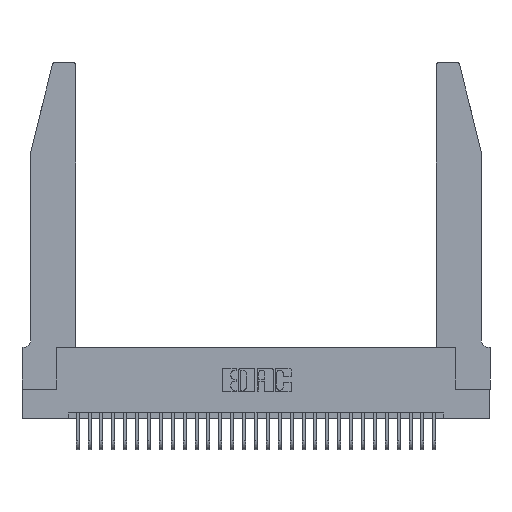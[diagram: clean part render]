
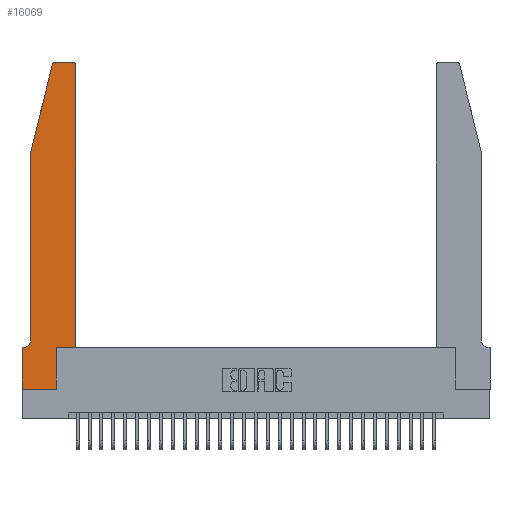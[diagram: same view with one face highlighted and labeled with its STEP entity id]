
A CAD part, top view. The second image highlights one B-rep face of the part: STEP entity #16069.
In plain terms, the highlighted planar face has unit normal (0, 0, 1).
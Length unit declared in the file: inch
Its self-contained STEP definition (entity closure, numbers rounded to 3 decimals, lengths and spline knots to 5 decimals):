
#297 = CARTESIAN_POINT ( 'NONE',  ( 0.4205, 2.72, 0.37 ) ) ;
#377 = EDGE_CURVE ( 'NONE', #8615, #3096, #2190, .T. ) ;
#385 = DIRECTION ( 'NONE',  ( 1., 0., 0. ) ) ;
#727 = EDGE_CURVE ( 'NONE', #26823, #5615, #28646, .T. ) ;
#1028 = EDGE_CURVE ( 'NONE', #5615, #10951, #1361, .T. ) ;
#1029 = CARTESIAN_POINT ( 'NONE',  ( 0.4505, 2.72, 0.37 ) ) ;
#1043 = VECTOR ( 'NONE', #2668, 39.37008 ) ;
#1126 = ORIENTED_EDGE ( 'NONE', *, *, #11851, .T. ) ;
#1361 = LINE ( 'NONE', #2361, #12913 ) ;
#1579 = EDGE_CURVE ( 'NONE', #10951, #21455, #11445, .T. ) ;
#1671 = CIRCLE ( 'NONE', #4736, 0.03 ) ;
#1751 = ORIENTED_EDGE ( 'NONE', *, *, #12945, .T. ) ;
#1956 = EDGE_LOOP ( 'NONE', ( #27631, #6244, #1751, #22483, #5915, #8851, #1126, #10419, #12542, #1984, #29123, #8060 ) ) ;
#1984 = ORIENTED_EDGE ( 'NONE', *, *, #727, .T. ) ;
#2190 = LINE ( 'NONE', #12530, #8380 ) ;
#2299 = VERTEX_POINT ( 'NONE', #7763 ) ;
#2361 = CARTESIAN_POINT ( 'NONE',  ( 0.4505, 0.35, 0.37 ) ) ;
#2425 = DIRECTION ( 'NONE',  ( 0., 0., -1. ) ) ;
#2523 = DIRECTION ( 'NONE',  ( 0., 1., 0. ) ) ;
#2608 = DIRECTION ( 'NONE',  ( 1., 0., 0. ) ) ;
#2668 = DIRECTION ( 'NONE',  ( -1., 0., 0. ) ) ;
#2748 = DIRECTION ( 'NONE',  ( 0., 0., 1. ) ) ;
#2757 = DIRECTION ( 'NONE',  ( 0., 1., 0. ) ) ;
#2860 = EDGE_CURVE ( 'NONE', #3096, #26823, #4192, .T. ) ;
#3047 = CARTESIAN_POINT ( 'NONE',  ( 0., 0.35, 0.37 ) ) ;
#3096 = VERTEX_POINT ( 'NONE', #26735 ) ;
#3155 = VECTOR ( 'NONE', #25083, 39.37008 ) ;
#3467 = CARTESIAN_POINT ( 'NONE',  ( 0.2865, 0.35, 0.37 ) ) ;
#3954 = LINE ( 'NONE', #26986, #15414 ) ;
#4134 = DIRECTION ( 'NONE',  ( 0., -1., 0. ) ) ;
#4192 = LINE ( 'NONE', #7428, #20300 ) ;
#4346 = CARTESIAN_POINT ( 'NONE',  ( 0., 0.35, 0.37 ) ) ;
#4482 = CARTESIAN_POINT ( 'NONE',  ( 0.2605, 2.75, 0.37 ) ) ;
#4736 = AXIS2_PLACEMENT_3D ( 'NONE', #16496, #2748, #18805 ) ;
#5313 = VECTOR ( 'NONE', #27944, 39.37008 ) ;
#5404 = VERTEX_POINT ( 'NONE', #3047 ) ;
#5615 = VERTEX_POINT ( 'NONE', #22076 ) ;
#5915 = ORIENTED_EDGE ( 'NONE', *, *, #7186, .T. ) ;
#6244 = ORIENTED_EDGE ( 'NONE', *, *, #22508, .T. ) ;
#6357 = DIRECTION ( 'NONE',  ( 0., -1., 0. ) ) ;
#6574 = EDGE_CURVE ( 'NONE', #11440, #5404, #14012, .T. ) ;
#7186 = EDGE_CURVE ( 'NONE', #2299, #11440, #21830, .T. ) ;
#7428 = CARTESIAN_POINT ( 'NONE',  ( 0.2865, 0.35, 0.37 ) ) ;
#7453 = CARTESIAN_POINT ( 'NONE',  ( 0.0755, 2., 0.37 ) ) ;
#7763 = CARTESIAN_POINT ( 'NONE',  ( 0.0755, 0.42, 0.37 ) ) ;
#8060 = ORIENTED_EDGE ( 'NONE', *, *, #1579, .T. ) ;
#8380 = VECTOR ( 'NONE', #385, 39.37008 ) ;
#8587 = FACE_OUTER_BOUND ( 'NONE', #1956, .T. ) ;
#8615 = VERTEX_POINT ( 'NONE', #10075 ) ;
#8851 = ORIENTED_EDGE ( 'NONE', *, *, #6574, .T. ) ;
#9110 = PLANE ( 'NONE',  #16142 ) ;
#9832 = CARTESIAN_POINT ( 'NONE',  ( 0.25487, 2.72718, 0.37 ) ) ;
#9971 = EDGE_CURVE ( 'NONE', #10111, #2299, #15187, .T. ) ;
#10066 = AXIS2_PLACEMENT_3D ( 'NONE', #16183, #2425, #18488 ) ;
#10075 = CARTESIAN_POINT ( 'NONE',  ( 0., 0., 0.37 ) ) ;
#10111 = VERTEX_POINT ( 'NONE', #13662 ) ;
#10419 = ORIENTED_EDGE ( 'NONE', *, *, #377, .T. ) ;
#10951 = VERTEX_POINT ( 'NONE', #1029 ) ;
#11294 = VECTOR ( 'NONE', #4134, 39.37008 ) ;
#11403 = DIRECTION ( 'NONE',  ( 0., 0., 1. ) ) ;
#11440 = VERTEX_POINT ( 'NONE', #14291 ) ;
#11445 = CIRCLE ( 'NONE', #16043, 0.03 ) ;
#11851 = EDGE_CURVE ( 'NONE', #5404, #8615, #3954, .T. ) ;
#12530 = CARTESIAN_POINT ( 'NONE',  ( 0., 0., 0.37 ) ) ;
#12542 = ORIENTED_EDGE ( 'NONE', *, *, #2860, .T. ) ;
#12600 = EDGE_CURVE ( 'NONE', #21455, #26869, #15356, .T. ) ;
#12913 = VECTOR ( 'NONE', #2523, 39.37008 ) ;
#12945 = EDGE_CURVE ( 'NONE', #21382, #10111, #23526, .T. ) ;
#13662 = CARTESIAN_POINT ( 'NONE',  ( 0.0755, 2., 0.37 ) ) ;
#14012 = LINE ( 'NONE', #21006, #1043 ) ;
#14291 = CARTESIAN_POINT ( 'NONE',  ( 0.0055, 0.35, 0.37 ) ) ;
#15187 = LINE ( 'NONE', #17863, #11294 ) ;
#15356 = LINE ( 'NONE', #4482, #3155 ) ;
#15414 = VECTOR ( 'NONE', #6357, 39.37008 ) ;
#15495 = CARTESIAN_POINT ( 'NONE',  ( 0.4505, 0.35, 0.37 ) ) ;
#16043 = AXIS2_PLACEMENT_3D ( 'NONE', #297, #16364, #2608 ) ;
#16069 = ADVANCED_FACE ( 'NONE', ( #8587 ), #9110, .T. ) ;
#16142 = AXIS2_PLACEMENT_3D ( 'NONE', #4346, #11403, #27275 ) ;
#16183 = CARTESIAN_POINT ( 'NONE',  ( 0.0055, 0.42, 0.37 ) ) ;
#16364 = DIRECTION ( 'NONE',  ( 0., 0., 1. ) ) ;
#16496 = CARTESIAN_POINT ( 'NONE',  ( 0.284, 2.72, 0.37 ) ) ;
#17863 = CARTESIAN_POINT ( 'NONE',  ( 0.0755, 2., 0.37 ) ) ;
#18488 = DIRECTION ( 'NONE',  ( -1., 0., 0. ) ) ;
#18805 = DIRECTION ( 'NONE',  ( 1., 0., 0. ) ) ;
#20300 = VECTOR ( 'NONE', #2757, 39.37008 ) ;
#21006 = CARTESIAN_POINT ( 'NONE',  ( 0.0755, 0.35, 0.37 ) ) ;
#21382 = VERTEX_POINT ( 'NONE', #9832 ) ;
#21455 = VERTEX_POINT ( 'NONE', #25897 ) ;
#21830 = CIRCLE ( 'NONE', #10066, 0.07 ) ;
#22076 = CARTESIAN_POINT ( 'NONE',  ( 0.4505, 0.35, 0.37 ) ) ;
#22483 = ORIENTED_EDGE ( 'NONE', *, *, #9971, .T. ) ;
#22508 = EDGE_CURVE ( 'NONE', #26869, #21382, #1671, .T. ) ;
#22604 = VECTOR ( 'NONE', #25224, 39.37008 ) ;
#23526 = LINE ( 'NONE', #7453, #5313 ) ;
#25083 = DIRECTION ( 'NONE',  ( -1., 0., 0. ) ) ;
#25224 = DIRECTION ( 'NONE',  ( 1., 0., 0. ) ) ;
#25897 = CARTESIAN_POINT ( 'NONE',  ( 0.4205, 2.75, 0.37 ) ) ;
#26735 = CARTESIAN_POINT ( 'NONE',  ( 0.2865, 0., 0.37 ) ) ;
#26823 = VERTEX_POINT ( 'NONE', #3467 ) ;
#26869 = VERTEX_POINT ( 'NONE', #28731 ) ;
#26986 = CARTESIAN_POINT ( 'NONE',  ( 0., 0., 0.37 ) ) ;
#27275 = DIRECTION ( 'NONE',  ( 1., 0., 0. ) ) ;
#27631 = ORIENTED_EDGE ( 'NONE', *, *, #12600, .T. ) ;
#27944 = DIRECTION ( 'NONE',  ( -0.239, -0.971, 0. ) ) ;
#28646 = LINE ( 'NONE', #15495, #22604 ) ;
#28731 = CARTESIAN_POINT ( 'NONE',  ( 0.284, 2.75, 0.37 ) ) ;
#29123 = ORIENTED_EDGE ( 'NONE', *, *, #1028, .T. ) ;
